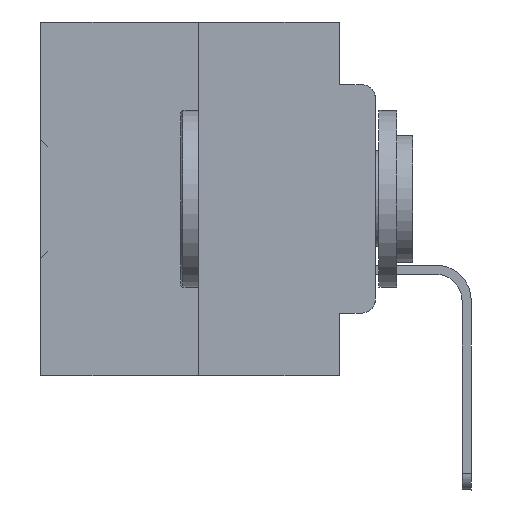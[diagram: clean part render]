
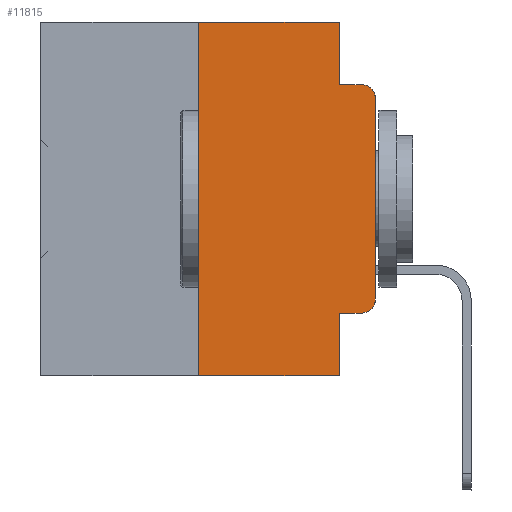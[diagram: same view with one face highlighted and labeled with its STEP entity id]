
A CAD part, left-side view. The second image highlights one B-rep face of the part: STEP entity #11815.
In plain terms, the highlighted planar face has unit normal (-1, 0, 0).
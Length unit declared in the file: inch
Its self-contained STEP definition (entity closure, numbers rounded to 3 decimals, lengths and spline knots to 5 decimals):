
#211 = CARTESIAN_POINT ( 'NONE',  ( 0., 0.25, 0. ) ) ;
#301 = DIRECTION ( 'NONE',  ( 0., 0., -1. ) ) ;
#441 = VECTOR ( 'NONE', #34284, 39.37008 ) ;
#1202 = LINE ( 'NONE', #12045, #12183 ) ;
#1680 = PLANE ( 'NONE',  #13844 ) ;
#2208 = ORIENTED_EDGE ( 'NONE', *, *, #8509, .F. ) ;
#2258 = LINE ( 'NONE', #26364, #5942 ) ;
#2586 = LINE ( 'NONE', #36102, #10379 ) ;
#3388 = CARTESIAN_POINT ( 'NONE',  ( 0., 0.473, 0. ) ) ;
#4274 = CARTESIAN_POINT ( 'NONE',  ( 0., 0.051, -0.4115 ) ) ;
#4308 = DIRECTION ( 'NONE',  ( 0., -1., 0. ) ) ;
#4616 = CARTESIAN_POINT ( 'NONE',  ( 0., 0.473, 0. ) ) ;
#4672 = LINE ( 'NONE', #3388, #15230 ) ;
#4870 = DIRECTION ( 'NONE',  ( 1., 0., 0. ) ) ;
#5368 = VERTEX_POINT ( 'NONE', #11618 ) ;
#5629 = VERTEX_POINT ( 'NONE', #15739 ) ;
#5942 = VECTOR ( 'NONE', #8834, 39.37008 ) ;
#6225 = EDGE_CURVE ( 'NONE', #22784, #33482, #14591, .T. ) ;
#6740 = AXIS2_PLACEMENT_3D ( 'NONE', #30010, #9626, #301 ) ;
#6787 = VECTOR ( 'NONE', #4308, 39.37008 ) ;
#7384 = DIRECTION ( 'NONE',  ( -1., 0., 0. ) ) ;
#7454 = DIRECTION ( 'NONE',  ( 0., 0., 1. ) ) ;
#7775 = ORIENTED_EDGE ( 'NONE', *, *, #6225, .T. ) ;
#8509 = EDGE_CURVE ( 'NONE', #5629, #20807, #1202, .T. ) ;
#8834 = DIRECTION ( 'NONE',  ( 0., -1., 0. ) ) ;
#9281 = DIRECTION ( 'NONE',  ( 0., -1., 0. ) ) ;
#9626 = DIRECTION ( 'NONE',  ( -1., 0., 0. ) ) ;
#10379 = VECTOR ( 'NONE', #7454, 39.37008 ) ;
#10440 = LINE ( 'NONE', #13890, #14101 ) ;
#11618 = CARTESIAN_POINT ( 'NONE',  ( 0., 0., -0.1085 ) ) ;
#11815 = ADVANCED_FACE ( 'NONE', ( #15182 ), #1680, .F. ) ;
#12045 = CARTESIAN_POINT ( 'NONE',  ( 0., 0.25, 0. ) ) ;
#12183 = VECTOR ( 'NONE', #29853, 39.37008 ) ;
#12547 = ORIENTED_EDGE ( 'NONE', *, *, #26022, .F. ) ;
#13023 = ORIENTED_EDGE ( 'NONE', *, *, #31172, .F. ) ;
#13073 = EDGE_LOOP ( 'NONE', ( #28125, #14416, #33192, #13023, #12547, #2208, #19836, #19869, #7775, #32084 ) ) ;
#13147 = CARTESIAN_POINT ( 'NONE',  ( 0., 0.051, -0.0885 ) ) ;
#13375 = VECTOR ( 'NONE', #33048, 39.37008 ) ;
#13571 = CARTESIAN_POINT ( 'NONE',  ( 0., 0.051, 0. ) ) ;
#13844 = AXIS2_PLACEMENT_3D ( 'NONE', #4616, #4870, #25474 ) ;
#13890 = CARTESIAN_POINT ( 'NONE',  ( 0., 0.051, -0.0885 ) ) ;
#14101 = VECTOR ( 'NONE', #16862, 39.37008 ) ;
#14416 = ORIENTED_EDGE ( 'NONE', *, *, #19109, .T. ) ;
#14591 = LINE ( 'NONE', #22118, #6787 ) ;
#15182 = FACE_OUTER_BOUND ( 'NONE', #13073, .T. ) ;
#15230 = VECTOR ( 'NONE', #9281, 39.37008 ) ;
#15739 = CARTESIAN_POINT ( 'NONE',  ( 0., 0.25, -0.5 ) ) ;
#16862 = DIRECTION ( 'NONE',  ( 0., -1., 0. ) ) ;
#17076 = CIRCLE ( 'NONE', #35927, 0.02 ) ;
#17619 = VERTEX_POINT ( 'NONE', #19853 ) ;
#17969 = CARTESIAN_POINT ( 'NONE',  ( 0., 0.051, 0. ) ) ;
#18782 = CARTESIAN_POINT ( 'NONE',  ( 0., 0.02, -0.3915 ) ) ;
#18892 = LINE ( 'NONE', #17969, #13375 ) ;
#19109 = EDGE_CURVE ( 'NONE', #5368, #27455, #30722, .T. ) ;
#19836 = ORIENTED_EDGE ( 'NONE', *, *, #21808, .T. ) ;
#19853 = CARTESIAN_POINT ( 'NONE',  ( 0., 0.051, -0.5 ) ) ;
#19869 = ORIENTED_EDGE ( 'NONE', *, *, #35281, .F. ) ;
#20397 = CARTESIAN_POINT ( 'NONE',  ( 0., 0.02, -0.4115 ) ) ;
#20420 = EDGE_CURVE ( 'NONE', #33482, #27897, #17076, .T. ) ;
#20807 = VERTEX_POINT ( 'NONE', #211 ) ;
#21808 = EDGE_CURVE ( 'NONE', #5629, #17619, #2258, .T. ) ;
#22118 = CARTESIAN_POINT ( 'NONE',  ( 0., 0.051, -0.4115 ) ) ;
#22146 = VERTEX_POINT ( 'NONE', #13147 ) ;
#22417 = EDGE_CURVE ( 'NONE', #22146, #27455, #10440, .T. ) ;
#22784 = VERTEX_POINT ( 'NONE', #4274 ) ;
#24305 = EDGE_CURVE ( 'NONE', #27897, #5368, #2586, .T. ) ;
#24929 = DIRECTION ( 'NONE',  ( 0., 0., -1. ) ) ;
#25165 = CARTESIAN_POINT ( 'NONE',  ( 0., 0.02, -0.0885 ) ) ;
#25474 = DIRECTION ( 'NONE',  ( 0., 0., -1. ) ) ;
#26022 = EDGE_CURVE ( 'NONE', #20807, #26341, #4672, .T. ) ;
#26341 = VERTEX_POINT ( 'NONE', #28314 ) ;
#26364 = CARTESIAN_POINT ( 'NONE',  ( 0., 0.473, -0.5 ) ) ;
#27455 = VERTEX_POINT ( 'NONE', #25165 ) ;
#27897 = VERTEX_POINT ( 'NONE', #35607 ) ;
#28125 = ORIENTED_EDGE ( 'NONE', *, *, #24305, .T. ) ;
#28314 = CARTESIAN_POINT ( 'NONE',  ( 0., 0.051, 0. ) ) ;
#29853 = DIRECTION ( 'NONE',  ( 0., 0., 1. ) ) ;
#30010 = CARTESIAN_POINT ( 'NONE',  ( 0., 0.02, -0.1085 ) ) ;
#30722 = CIRCLE ( 'NONE', #6740, 0.02 ) ;
#31172 = EDGE_CURVE ( 'NONE', #26341, #22146, #18892, .T. ) ;
#32069 = LINE ( 'NONE', #13571, #441 ) ;
#32084 = ORIENTED_EDGE ( 'NONE', *, *, #20420, .T. ) ;
#33048 = DIRECTION ( 'NONE',  ( 0., 0., -1. ) ) ;
#33192 = ORIENTED_EDGE ( 'NONE', *, *, #22417, .F. ) ;
#33482 = VERTEX_POINT ( 'NONE', #20397 ) ;
#34284 = DIRECTION ( 'NONE',  ( 0., 0., -1. ) ) ;
#35281 = EDGE_CURVE ( 'NONE', #22784, #17619, #32069, .T. ) ;
#35607 = CARTESIAN_POINT ( 'NONE',  ( 0., 0., -0.3915 ) ) ;
#35927 = AXIS2_PLACEMENT_3D ( 'NONE', #18782, #7384, #24929 ) ;
#36102 = CARTESIAN_POINT ( 'NONE',  ( 0., 0., 0. ) ) ;
